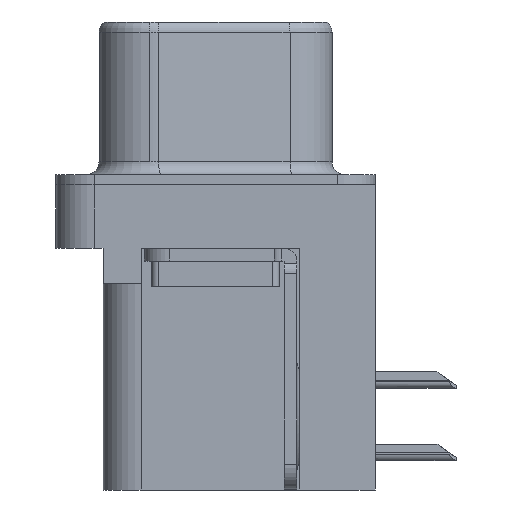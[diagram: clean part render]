
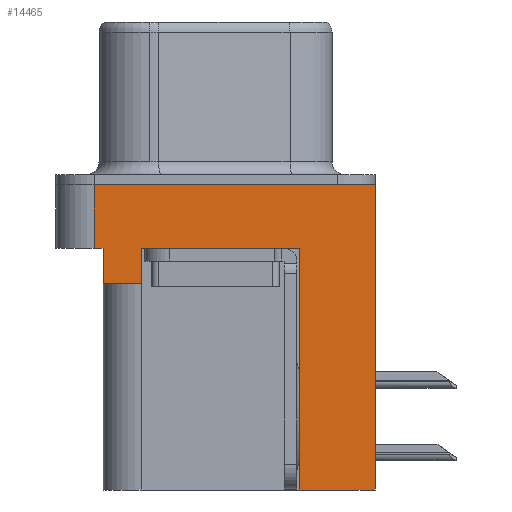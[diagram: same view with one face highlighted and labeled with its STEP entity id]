
A CAD part, left-side view. The second image highlights one B-rep face of the part: STEP entity #14465.
In plain terms, the highlighted planar face has unit normal (-1, 0, 0).
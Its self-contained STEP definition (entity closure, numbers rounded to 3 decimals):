
#676 = ORIENTED_EDGE ( 'NONE', *, *, #21055, .F. ) ;
#940 = VECTOR ( 'NONE', #5598, 1000. ) ;
#1341 = DIRECTION ( 'NONE',  ( 0., 1., 0. ) ) ;
#1578 = EDGE_CURVE ( 'NONE', #14210, #11507, #7395, .T. ) ;
#2373 = ORIENTED_EDGE ( 'NONE', *, *, #13790, .F. ) ;
#2428 = AXIS2_PLACEMENT_3D ( 'NONE', #8016, #6082, #7879 ) ;
#2463 = VECTOR ( 'NONE', #1341, 1000. ) ;
#2798 = LINE ( 'NONE', #17029, #14303 ) ;
#2895 = ORIENTED_EDGE ( 'NONE', *, *, #13546, .F. ) ;
#3371 = LINE ( 'NONE', #6553, #16464 ) ;
#3855 = VERTEX_POINT ( 'NONE', #18779 ) ;
#4843 = DIRECTION ( 'NONE',  ( 0., 0., 1. ) ) ;
#4927 = CARTESIAN_POINT ( 'NONE',  ( -3., -6.275, 0. ) ) ;
#4955 = DIRECTION ( 'NONE',  ( 0., 0., 1. ) ) ;
#5224 = VERTEX_POINT ( 'NONE', #7094 ) ;
#5517 = DIRECTION ( 'NONE',  ( 0., -1., 0. ) ) ;
#5598 = DIRECTION ( 'NONE',  ( 0., -1., 0. ) ) ;
#5648 = LINE ( 'NONE', #7231, #6966 ) ;
#5876 = EDGE_CURVE ( 'NONE', #15949, #15097, #14710, .T. ) ;
#6082 = DIRECTION ( 'NONE',  ( -1., 0., 0. ) ) ;
#6553 = CARTESIAN_POINT ( 'NONE',  ( -3., -3.295, -12. ) ) ;
#6773 = CARTESIAN_POINT ( 'NONE',  ( -3., -6.275, 0. ) ) ;
#6966 = VECTOR ( 'NONE', #8945, 1000. ) ;
#7084 = LINE ( 'NONE', #12225, #940 ) ;
#7094 = CARTESIAN_POINT ( 'NONE',  ( -3., -6.275, -12. ) ) ;
#7192 = VERTEX_POINT ( 'NONE', #18013 ) ;
#7231 = CARTESIAN_POINT ( 'NONE',  ( -3., -6.275, -2.5 ) ) ;
#7317 = EDGE_CURVE ( 'NONE', #12051, #11507, #3371, .T. ) ;
#7395 = LINE ( 'NONE', #20132, #15679 ) ;
#7409 = VERTEX_POINT ( 'NONE', #6773 ) ;
#7775 = LINE ( 'NONE', #16503, #21694 ) ;
#7879 = DIRECTION ( 'NONE',  ( 0., 0., 1. ) ) ;
#8016 = CARTESIAN_POINT ( 'NONE',  ( -3., -6.275, -2.5 ) ) ;
#8289 = FACE_OUTER_BOUND ( 'NONE', #13213, .T. ) ;
#8945 = DIRECTION ( 'NONE',  ( 0., 0., 1. ) ) ;
#10576 = CARTESIAN_POINT ( 'NONE',  ( -3., 4.425, -3.9 ) ) ;
#10934 = CARTESIAN_POINT ( 'NONE',  ( -3., 2.895, -3.9 ) ) ;
#11240 = PLANE ( 'NONE',  #2428 ) ;
#11275 = LINE ( 'NONE', #10576, #2463 ) ;
#11341 = DIRECTION ( 'NONE',  ( 0., 1., 0. ) ) ;
#11507 = VERTEX_POINT ( 'NONE', #18910 ) ;
#11843 = DIRECTION ( 'NONE',  ( 0., 0., 1. ) ) ;
#12036 = LINE ( 'NONE', #4927, #17668 ) ;
#12051 = VERTEX_POINT ( 'NONE', #18664 ) ;
#12225 = CARTESIAN_POINT ( 'NONE',  ( -3., -6.275, -2.5 ) ) ;
#12494 = ORIENTED_EDGE ( 'NONE', *, *, #7317, .F. ) ;
#13023 = DIRECTION ( 'NONE',  ( 0., 0., 1. ) ) ;
#13213 = EDGE_LOOP ( 'NONE', ( #17393, #676, #13247, #20992, #2895, #20758, #21632, #12494, #2373, #17721 ) ) ;
#13247 = ORIENTED_EDGE ( 'NONE', *, *, #21207, .T. ) ;
#13546 = EDGE_CURVE ( 'NONE', #15832, #15949, #11275, .T. ) ;
#13790 = EDGE_CURVE ( 'NONE', #5224, #12051, #7775, .T. ) ;
#13899 = LINE ( 'NONE', #19621, #18189 ) ;
#14186 = EDGE_CURVE ( 'NONE', #5224, #7409, #5648, .T. ) ;
#14210 = VERTEX_POINT ( 'NONE', #15915 ) ;
#14303 = VECTOR ( 'NONE', #11843, 1000. ) ;
#14465 = ADVANCED_FACE ( 'NONE', ( #8289 ), #11240, .T. ) ;
#14710 = LINE ( 'NONE', #14895, #15537 ) ;
#14783 = CARTESIAN_POINT ( 'NONE',  ( -3., 4.425, -3.9 ) ) ;
#14895 = CARTESIAN_POINT ( 'NONE',  ( -3., 4.425, -3.9 ) ) ;
#14978 = DIRECTION ( 'NONE',  ( 0., -1., 0. ) ) ;
#15097 = VERTEX_POINT ( 'NONE', #16308 ) ;
#15537 = VECTOR ( 'NONE', #13023, 1000. ) ;
#15679 = VECTOR ( 'NONE', #14978, 1000. ) ;
#15832 = VERTEX_POINT ( 'NONE', #10934 ) ;
#15915 = CARTESIAN_POINT ( 'NONE',  ( -3., 2.895, -2.5 ) ) ;
#15949 = VERTEX_POINT ( 'NONE', #14783 ) ;
#16308 = CARTESIAN_POINT ( 'NONE',  ( -3., 4.425, -2.5 ) ) ;
#16464 = VECTOR ( 'NONE', #4843, 1000. ) ;
#16503 = CARTESIAN_POINT ( 'NONE',  ( -3., -3.295, -12. ) ) ;
#17029 = CARTESIAN_POINT ( 'NONE',  ( -3., 4.775, -2.5 ) ) ;
#17393 = ORIENTED_EDGE ( 'NONE', *, *, #22089, .F. ) ;
#17668 = VECTOR ( 'NONE', #5517, 1000. ) ;
#17721 = ORIENTED_EDGE ( 'NONE', *, *, #14186, .T. ) ;
#18013 = CARTESIAN_POINT ( 'NONE',  ( -3., 4.775, -2.5 ) ) ;
#18189 = VECTOR ( 'NONE', #4955, 1000. ) ;
#18664 = CARTESIAN_POINT ( 'NONE',  ( -3., -3.295, -12. ) ) ;
#18779 = CARTESIAN_POINT ( 'NONE',  ( -3., 4.775, 0. ) ) ;
#18910 = CARTESIAN_POINT ( 'NONE',  ( -3., -3.295, -2.5 ) ) ;
#19621 = CARTESIAN_POINT ( 'NONE',  ( -3., 2.895, -3.9 ) ) ;
#20132 = CARTESIAN_POINT ( 'NONE',  ( -3., -6.275, -2.5 ) ) ;
#20758 = ORIENTED_EDGE ( 'NONE', *, *, #22021, .T. ) ;
#20992 = ORIENTED_EDGE ( 'NONE', *, *, #5876, .F. ) ;
#21055 = EDGE_CURVE ( 'NONE', #7192, #3855, #2798, .T. ) ;
#21207 = EDGE_CURVE ( 'NONE', #7192, #15097, #7084, .T. ) ;
#21632 = ORIENTED_EDGE ( 'NONE', *, *, #1578, .T. ) ;
#21694 = VECTOR ( 'NONE', #11341, 1000. ) ;
#22021 = EDGE_CURVE ( 'NONE', #15832, #14210, #13899, .T. ) ;
#22089 = EDGE_CURVE ( 'NONE', #3855, #7409, #12036, .T. ) ;
